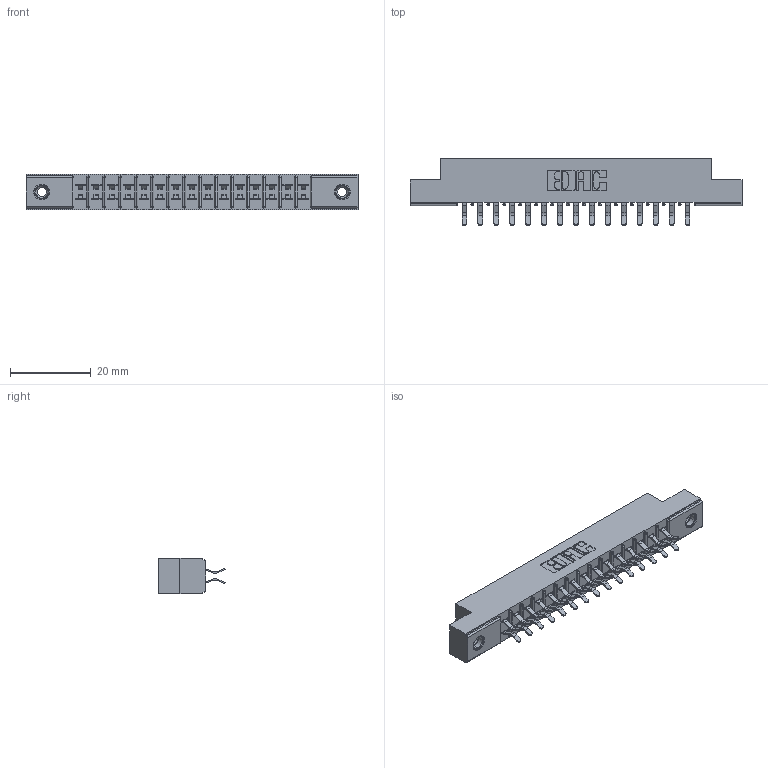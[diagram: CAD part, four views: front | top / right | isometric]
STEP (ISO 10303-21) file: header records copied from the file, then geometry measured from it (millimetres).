
FILE_DESCRIPTION (( 'STEP AP203' ), '1' );
FILE_NAME ('355-030-556-508.STEP', '2019-09-11T07:31:58', ( '' ), ( '' ), 'SwSTEP 2.0', 'SolidWorks 2016', '' );
FILE_SCHEMA (( 'CONFIG_CONTROL_DESIGN' ));
Length unit declared in the file: inch
Products named in the file (4): 345-250-001_345-250-003-102; 305-290-001_556; 355-030-556-508; 305 Part_.156 Dia
Assembly tree (33 placements, depth 2):
  355-030-556-508
    305 Part_.156 Dia
    305-290-001_556  x30
    345-250-001_345-250-003-102  x2
Bounding box: 82.45 x 16.64 x 8.71 mm (x, y, z)
Volume: 4957.3 mm3; surface area: 9462.3 mm2
Topology: 33 solids, 33 shells, 1856 faces, 5297 edges, 3442 vertices
Faces by surface type: plane 1030, cylinder 750, sphere 60, cone 12, torus 4
Entity records: 20935 total; most frequent: CARTESIAN_POINT 3450, ORIENTED_EDGE 3414, DIRECTION 3373, EDGE_CURVE 1707, LINE 1343, VECTOR 1343, VERTEX_POINT 1092, AXIS2_PLACEMENT_3D 1015
